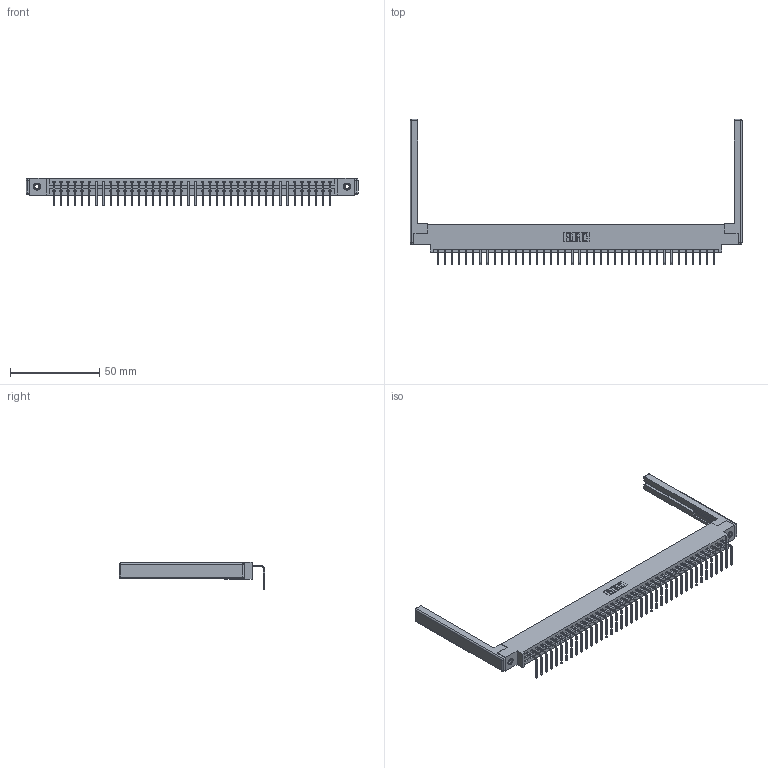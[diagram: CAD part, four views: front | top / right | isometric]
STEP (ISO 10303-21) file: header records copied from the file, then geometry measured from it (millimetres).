
FILE_DESCRIPTION (( 'STEP AP203' ), '1' );
FILE_NAME ('387-040-558-668.STEP', '2019-10-07T21:32:26', ( '' ), ( '' ), 'SwSTEP 2.0', 'SolidWorks 2016', '' );
FILE_SCHEMA (( 'CONFIG_CONTROL_DESIGN' ));
Length unit declared in the file: inch
Products named in the file (5): 387-040-558-668; 337 Part_0.170 Offset - 0.156 Dia-TI; 345-250-001_345-250-001-102; 307-220-068; 345-292-001_558 Tail - 2
Assembly tree (45 placements, depth 2):
  387-040-558-668
    337 Part_0.170 Offset - 0.156 Dia-TI
    345-292-001_558 Tail - 2  x40
    345-250-001_345-250-001-102  x2
    307-220-068  x2
Bounding box: 185.93 x 81.22 x 15.37 mm (x, y, z)
Volume: 23706.1 mm3; surface area: 24955.8 mm2
Topology: 45 solids, 45 shells, 2832 faces, 8473 edges, 5574 vertices
Faces by surface type: plane 2082, cylinder 726, cone 12, sphere 8, torus 4
Entity records: 32968 total; most frequent: CARTESIAN_POINT 5699, ORIENTED_EDGE 5664, DIRECTION 4874, EDGE_CURVE 2832, LINE 2654, VECTOR 2654, VERTEX_POINT 1878, AXIS2_PLACEMENT_3D 1110
